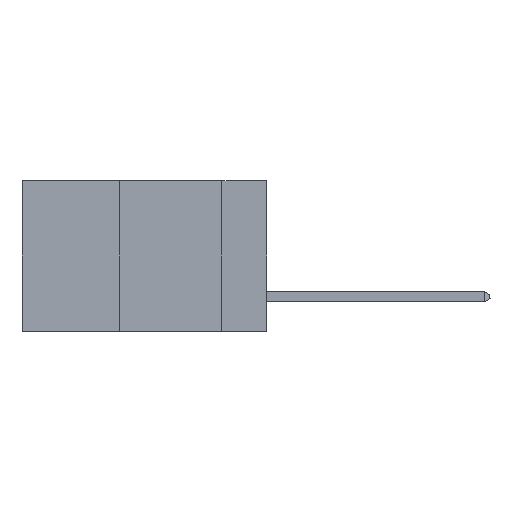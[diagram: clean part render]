
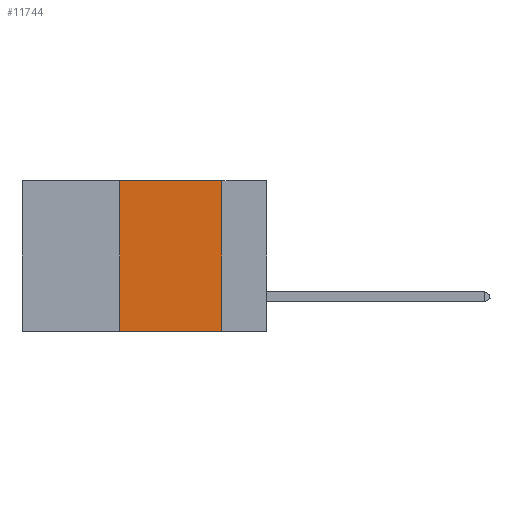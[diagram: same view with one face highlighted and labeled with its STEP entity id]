
A CAD part, left-side view. The second image highlights one B-rep face of the part: STEP entity #11744.
In plain terms, the highlighted planar face has unit normal (-1, 0, 0).
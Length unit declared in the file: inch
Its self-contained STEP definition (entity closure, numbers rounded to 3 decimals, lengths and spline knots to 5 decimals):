
#692 = VECTOR ( 'NONE', #42558, 39.37008 ) ;
#743 = LINE ( 'NONE', #5301, #15657 ) ;
#1575 = EDGE_CURVE ( 'NONE', #9399, #13447, #41323, .T. ) ;
#3507 = CARTESIAN_POINT ( 'NONE',  ( 0., 0.36, 0. ) ) ;
#5301 = CARTESIAN_POINT ( 'NONE',  ( 0., 0.11, 0. ) ) ;
#5974 = LINE ( 'NONE', #27137, #22390 ) ;
#6387 = DIRECTION ( 'NONE',  ( 0., 0., 1. ) ) ;
#6973 = EDGE_CURVE ( 'NONE', #11481, #30308, #13243, .T. ) ;
#6976 = CARTESIAN_POINT ( 'NONE',  ( 0., 0.6, 0. ) ) ;
#9399 = VERTEX_POINT ( 'NONE', #3507 ) ;
#11481 = VERTEX_POINT ( 'NONE', #28575 ) ;
#11744 = ADVANCED_FACE ( 'NONE', ( #28478 ), #34237, .F. ) ;
#13243 = LINE ( 'NONE', #23659, #41455 ) ;
#13435 = ORIENTED_EDGE ( 'NONE', *, *, #37240, .F. ) ;
#13447 = VERTEX_POINT ( 'NONE', #36165 ) ;
#15654 = CARTESIAN_POINT ( 'NONE',  ( 0., 0.6, 0. ) ) ;
#15657 = VECTOR ( 'NONE', #22185, 39.37008 ) ;
#19448 = EDGE_CURVE ( 'NONE', #13447, #30308, #743, .T. ) ;
#21637 = ORIENTED_EDGE ( 'NONE', *, *, #1575, .F. ) ;
#22185 = DIRECTION ( 'NONE',  ( 0., 0., -1. ) ) ;
#22390 = VECTOR ( 'NONE', #6387, 39.37008 ) ;
#23659 = CARTESIAN_POINT ( 'NONE',  ( 0., 0.6, -0.37 ) ) ;
#26007 = CARTESIAN_POINT ( 'NONE',  ( 0., 0.11, -0.37 ) ) ;
#26247 = ORIENTED_EDGE ( 'NONE', *, *, #6973, .T. ) ;
#26898 = DIRECTION ( 'NONE',  ( 1., 0., 0. ) ) ;
#27137 = CARTESIAN_POINT ( 'NONE',  ( 0., 0.36, 0. ) ) ;
#27412 = DIRECTION ( 'NONE',  ( 0., -1., 0. ) ) ;
#28478 = FACE_OUTER_BOUND ( 'NONE', #37625, .T. ) ;
#28575 = CARTESIAN_POINT ( 'NONE',  ( 0., 0.36, -0.37 ) ) ;
#30308 = VERTEX_POINT ( 'NONE', #26007 ) ;
#32293 = ORIENTED_EDGE ( 'NONE', *, *, #19448, .F. ) ;
#34237 = PLANE ( 'NONE',  #41435 ) ;
#36165 = CARTESIAN_POINT ( 'NONE',  ( 0., 0.11, 0. ) ) ;
#37240 = EDGE_CURVE ( 'NONE', #11481, #9399, #5974, .T. ) ;
#37625 = EDGE_LOOP ( 'NONE', ( #32293, #21637, #13435, #26247 ) ) ;
#37650 = DIRECTION ( 'NONE',  ( 0., 0., -1. ) ) ;
#41323 = LINE ( 'NONE', #15654, #692 ) ;
#41435 = AXIS2_PLACEMENT_3D ( 'NONE', #6976, #26898, #37650 ) ;
#41455 = VECTOR ( 'NONE', #27412, 39.37008 ) ;
#42558 = DIRECTION ( 'NONE',  ( 0., -1., 0. ) ) ;
